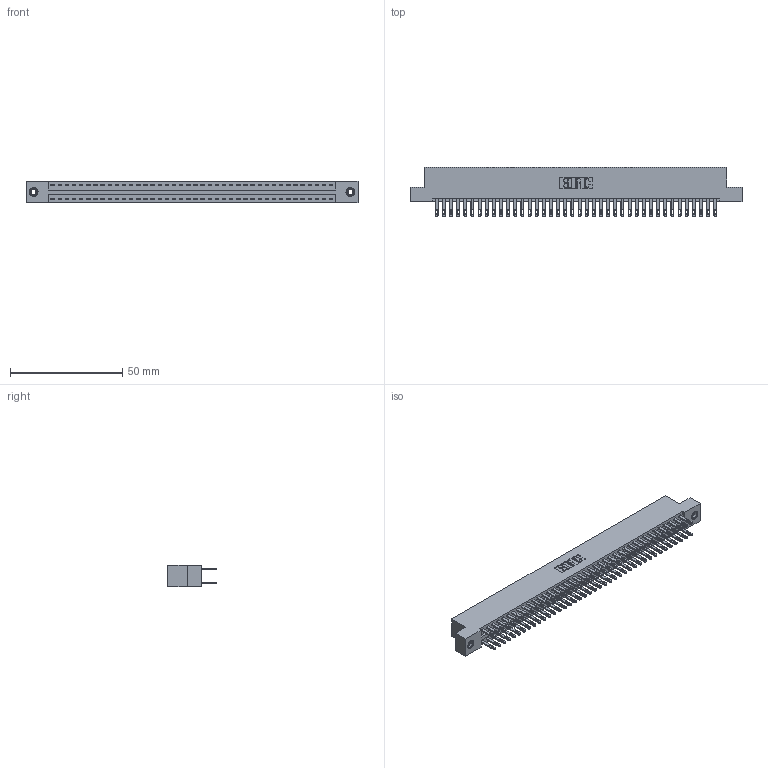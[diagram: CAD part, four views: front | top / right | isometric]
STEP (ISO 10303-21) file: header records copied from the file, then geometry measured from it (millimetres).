
FILE_DESCRIPTION (( 'STEP AP203' ), '1' );
FILE_NAME ('346-080-500-208.STEP', '2018-08-29T06:52:09', ( '' ), ( '' ), 'SwSTEP 2.0', 'SolidWorks 2016', '' );
FILE_SCHEMA (( 'CONFIG_CONTROL_DESIGN' ));
Length unit declared in the file: inch
Products named in the file (4): 345-250-001_345-250-003-102; 346-080-500-208; 346 Part_Flush Mounting Lugs - 0.156 Dia-TI; 345-292-001_345-293-100
Assembly tree (83 placements, depth 2):
  346-080-500-208
    346 Part_Flush Mounting Lugs - 0.156 Dia-TI
    345-292-001_345-293-100  x80
    345-250-001_345-250-003-102  x2
Bounding box: 147.57 x 21.84 x 9.4 mm (x, y, z)
Volume: 14612.7 mm3; surface area: 20912.1 mm2
Topology: 83 solids, 83 shells, 4022 faces, 12225 edges, 8142 vertices
Faces by surface type: plane 2428, cylinder 1578, cone 12, torus 4
Entity records: 27490 total; most frequent: CARTESIAN_POINT 4515, ORIENTED_EDGE 4442, DIRECTION 4059, EDGE_CURVE 2221, VECTOR 1905, LINE 1905, VERTEX_POINT 1476, AXIS2_PLACEMENT_3D 1077
